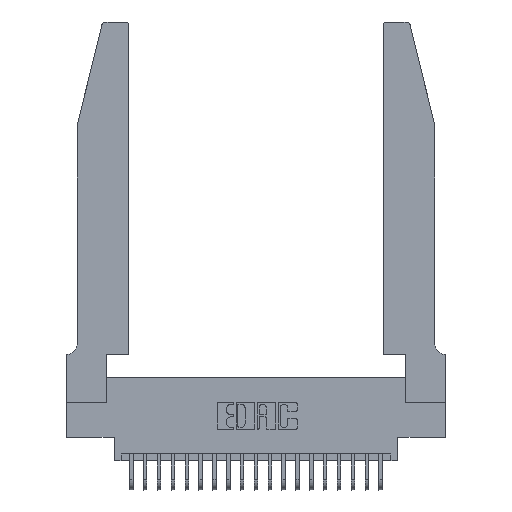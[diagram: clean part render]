
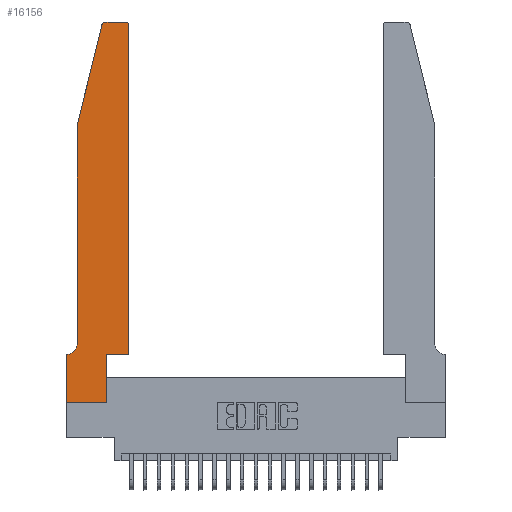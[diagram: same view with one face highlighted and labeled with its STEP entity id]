
A CAD part, top view. The second image highlights one B-rep face of the part: STEP entity #16156.
In plain terms, the highlighted planar face has unit normal (0, 0, 1).
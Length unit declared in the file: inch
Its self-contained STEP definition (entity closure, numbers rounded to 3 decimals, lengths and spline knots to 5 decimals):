
#381 = DIRECTION ( 'NONE',  ( 1., 0., 0. ) ) ;
#408 = VERTEX_POINT ( 'NONE', #17508 ) ;
#606 = AXIS2_PLACEMENT_3D ( 'NONE', #12163, #3018, #21847 ) ;
#843 = EDGE_CURVE ( 'NONE', #8329, #408, #15106, .T. ) ;
#1438 = VECTOR ( 'NONE', #5368, 39.37008 ) ;
#1468 = CARTESIAN_POINT ( 'NONE',  ( 0.0755, 2., 0.37 ) ) ;
#1613 = VERTEX_POINT ( 'NONE', #11266 ) ;
#1952 = ORIENTED_EDGE ( 'NONE', *, *, #3960, .T. ) ;
#2136 = CIRCLE ( 'NONE', #12913, 0.03 ) ;
#2166 = VERTEX_POINT ( 'NONE', #23242 ) ;
#2319 = CARTESIAN_POINT ( 'NONE',  ( 0.0755, 0.35, 0.37 ) ) ;
#2578 = LINE ( 'NONE', #14250, #4372 ) ;
#2602 = EDGE_LOOP ( 'NONE', ( #19045, #15794, #22098, #10497, #1952, #12947, #14258, #8536, #18576, #20081, #17790, #6834 ) ) ;
#2817 = CARTESIAN_POINT ( 'NONE',  ( 0.0055, 0.35, 0.37 ) ) ;
#3018 = DIRECTION ( 'NONE',  ( 0., 0., -1. ) ) ;
#3318 = EDGE_CURVE ( 'NONE', #7426, #1613, #6419, .T. ) ;
#3766 = DIRECTION ( 'NONE',  ( 0., 0., 1. ) ) ;
#3960 = EDGE_CURVE ( 'NONE', #1613, #8329, #13199, .T. ) ;
#4188 = AXIS2_PLACEMENT_3D ( 'NONE', #13577, #11826, #13739 ) ;
#4275 = VECTOR ( 'NONE', #8314, 39.37008 ) ;
#4372 = VECTOR ( 'NONE', #8711, 39.37008 ) ;
#4917 = VECTOR ( 'NONE', #21100, 39.37008 ) ;
#5160 = CARTESIAN_POINT ( 'NONE',  ( 0.4205, 2.75, 0.37 ) ) ;
#5257 = EDGE_CURVE ( 'NONE', #408, #17992, #16996, .T. ) ;
#5368 = DIRECTION ( 'NONE',  ( -0.239, -0.971, 0. ) ) ;
#5736 = CARTESIAN_POINT ( 'NONE',  ( 0.4205, 2.72, 0.37 ) ) ;
#5805 = VECTOR ( 'NONE', #8778, 39.37008 ) ;
#5874 = VECTOR ( 'NONE', #21283, 39.37008 ) ;
#6419 = LINE ( 'NONE', #19661, #4275 ) ;
#6482 = LINE ( 'NONE', #1468, #1438 ) ;
#6736 = DIRECTION ( 'NONE',  ( 0., 0., 1. ) ) ;
#6834 = ORIENTED_EDGE ( 'NONE', *, *, #12368, .T. ) ;
#7426 = VERTEX_POINT ( 'NONE', #8097 ) ;
#7586 = LINE ( 'NONE', #11561, #4917 ) ;
#8012 = CARTESIAN_POINT ( 'NONE',  ( 0., 0., 0.37 ) ) ;
#8097 = CARTESIAN_POINT ( 'NONE',  ( 0.0755, 2., 0.37 ) ) ;
#8229 = VECTOR ( 'NONE', #381, 39.37008 ) ;
#8314 = DIRECTION ( 'NONE',  ( 0., -1., 0. ) ) ;
#8329 = VERTEX_POINT ( 'NONE', #2817 ) ;
#8536 = ORIENTED_EDGE ( 'NONE', *, *, #16134, .T. ) ;
#8660 = DIRECTION ( 'NONE',  ( 1., 0., 0. ) ) ;
#8711 = DIRECTION ( 'NONE',  ( 0., 1., 0. ) ) ;
#8778 = DIRECTION ( 'NONE',  ( 1., 0., 0. ) ) ;
#9059 = VERTEX_POINT ( 'NONE', #16865 ) ;
#9140 = CARTESIAN_POINT ( 'NONE',  ( 0., 0., 0.37 ) ) ;
#10047 = EDGE_CURVE ( 'NONE', #14960, #18762, #7586, .T. ) ;
#10052 = LINE ( 'NONE', #11756, #5874 ) ;
#10056 = VECTOR ( 'NONE', #19537, 39.37008 ) ;
#10497 = ORIENTED_EDGE ( 'NONE', *, *, #3318, .T. ) ;
#10917 = CARTESIAN_POINT ( 'NONE',  ( 0.2865, 0.35, 0.37 ) ) ;
#11266 = CARTESIAN_POINT ( 'NONE',  ( 0.0755, 0.42, 0.37 ) ) ;
#11561 = CARTESIAN_POINT ( 'NONE',  ( 0.2865, 0.35, 0.37 ) ) ;
#11756 = CARTESIAN_POINT ( 'NONE',  ( 0.2605, 2.75, 0.37 ) ) ;
#11826 = DIRECTION ( 'NONE',  ( 0., 0., 1. ) ) ;
#12041 = LINE ( 'NONE', #13945, #5805 ) ;
#12163 = CARTESIAN_POINT ( 'NONE',  ( 0.0055, 0.42, 0.37 ) ) ;
#12368 = EDGE_CURVE ( 'NONE', #15519, #19922, #19900, .T. ) ;
#12586 = VERTEX_POINT ( 'NONE', #21424 ) ;
#12626 = CARTESIAN_POINT ( 'NONE',  ( 0.2865, 0., 0.37 ) ) ;
#12913 = AXIS2_PLACEMENT_3D ( 'NONE', #17753, #6736, #8660 ) ;
#12947 = ORIENTED_EDGE ( 'NONE', *, *, #843, .T. ) ;
#12996 = FACE_OUTER_BOUND ( 'NONE', #2602, .T. ) ;
#13199 = CIRCLE ( 'NONE', #606, 0.07 ) ;
#13577 = CARTESIAN_POINT ( 'NONE',  ( 0., 0.35, 0.37 ) ) ;
#13739 = DIRECTION ( 'NONE',  ( 1., 0., 0. ) ) ;
#13864 = LINE ( 'NONE', #8012, #8229 ) ;
#13945 = CARTESIAN_POINT ( 'NONE',  ( 0.4505, 0.35, 0.37 ) ) ;
#14250 = CARTESIAN_POINT ( 'NONE',  ( 0.4505, 0.35, 0.37 ) ) ;
#14258 = ORIENTED_EDGE ( 'NONE', *, *, #5257, .T. ) ;
#14300 = CARTESIAN_POINT ( 'NONE',  ( 0., 0., 0.37 ) ) ;
#14392 = DIRECTION ( 'NONE',  ( 0., -1., 0. ) ) ;
#14675 = EDGE_CURVE ( 'NONE', #19922, #12586, #10052, .T. ) ;
#14960 = VERTEX_POINT ( 'NONE', #12626 ) ;
#15106 = LINE ( 'NONE', #2319, #10056 ) ;
#15416 = PLANE ( 'NONE',  #4188 ) ;
#15519 = VERTEX_POINT ( 'NONE', #21778 ) ;
#15794 = ORIENTED_EDGE ( 'NONE', *, *, #23730, .T. ) ;
#16134 = EDGE_CURVE ( 'NONE', #17992, #14960, #13864, .T. ) ;
#16156 = ADVANCED_FACE ( 'NONE', ( #12996 ), #15416, .T. ) ;
#16865 = CARTESIAN_POINT ( 'NONE',  ( 0.25487, 2.72718, 0.37 ) ) ;
#16996 = LINE ( 'NONE', #14300, #20223 ) ;
#17358 = EDGE_CURVE ( 'NONE', #18762, #2166, #12041, .T. ) ;
#17508 = CARTESIAN_POINT ( 'NONE',  ( 0., 0.35, 0.37 ) ) ;
#17753 = CARTESIAN_POINT ( 'NONE',  ( 0.284, 2.72, 0.37 ) ) ;
#17790 = ORIENTED_EDGE ( 'NONE', *, *, #22716, .T. ) ;
#17992 = VERTEX_POINT ( 'NONE', #9140 ) ;
#18576 = ORIENTED_EDGE ( 'NONE', *, *, #10047, .T. ) ;
#18762 = VERTEX_POINT ( 'NONE', #10917 ) ;
#19045 = ORIENTED_EDGE ( 'NONE', *, *, #14675, .T. ) ;
#19537 = DIRECTION ( 'NONE',  ( -1., 0., 0. ) ) ;
#19661 = CARTESIAN_POINT ( 'NONE',  ( 0.0755, 2., 0.37 ) ) ;
#19900 = CIRCLE ( 'NONE', #23823, 0.03 ) ;
#19922 = VERTEX_POINT ( 'NONE', #5160 ) ;
#20081 = ORIENTED_EDGE ( 'NONE', *, *, #17358, .T. ) ;
#20223 = VECTOR ( 'NONE', #14392, 39.37008 ) ;
#21100 = DIRECTION ( 'NONE',  ( 0., 1., 0. ) ) ;
#21283 = DIRECTION ( 'NONE',  ( -1., 0., 0. ) ) ;
#21424 = CARTESIAN_POINT ( 'NONE',  ( 0.284, 2.75, 0.37 ) ) ;
#21778 = CARTESIAN_POINT ( 'NONE',  ( 0.4505, 2.72, 0.37 ) ) ;
#21847 = DIRECTION ( 'NONE',  ( -1., 0., 0. ) ) ;
#22098 = ORIENTED_EDGE ( 'NONE', *, *, #22797, .T. ) ;
#22716 = EDGE_CURVE ( 'NONE', #2166, #15519, #2578, .T. ) ;
#22797 = EDGE_CURVE ( 'NONE', #9059, #7426, #6482, .T. ) ;
#23018 = DIRECTION ( 'NONE',  ( 1., 0., 0. ) ) ;
#23242 = CARTESIAN_POINT ( 'NONE',  ( 0.4505, 0.35, 0.37 ) ) ;
#23730 = EDGE_CURVE ( 'NONE', #12586, #9059, #2136, .T. ) ;
#23823 = AXIS2_PLACEMENT_3D ( 'NONE', #5736, #3766, #23018 ) ;
